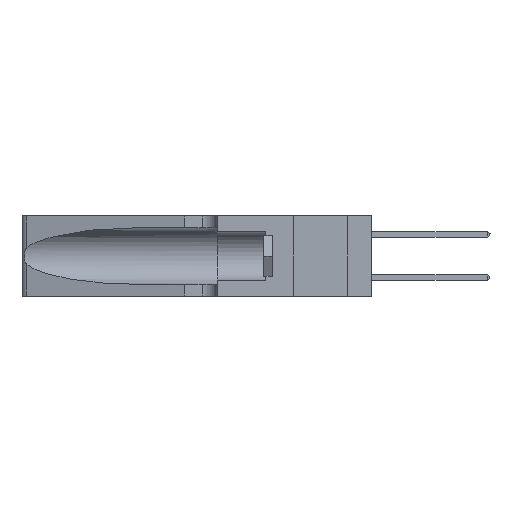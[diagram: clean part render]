
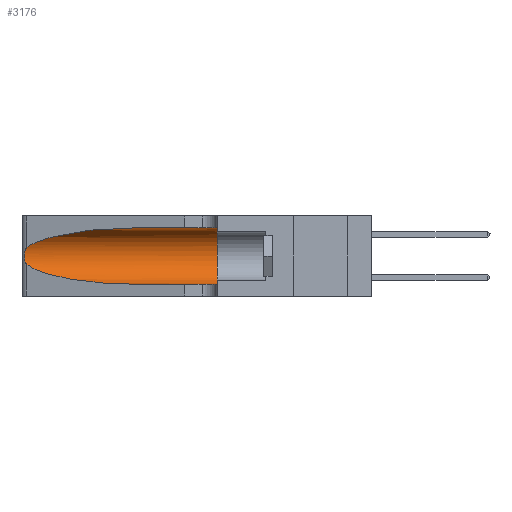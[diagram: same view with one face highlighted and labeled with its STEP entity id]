
A CAD part, left-side view. The second image highlights one B-rep face of the part: STEP entity #3176.
In plain terms, the highlighted cylindrical face has radius 3.308 mm (diameter 6.617 mm), a partial arc.
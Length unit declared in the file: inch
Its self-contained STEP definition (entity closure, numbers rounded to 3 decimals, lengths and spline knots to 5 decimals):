
#1540 = CARTESIAN_POINT ( 'NONE',  ( 0.25789, 1.23486, 0.15765 ) ) ;
#2517 = CARTESIAN_POINT ( 'NONE',  ( 0.1305, 1.61858, 0.185 ) ) ;
#3176 = ADVANCED_FACE ( 'NONE', ( #25702 ), #9307, .F. ) ;
#3346 =( BOUNDED_CURVE ( )  B_SPLINE_CURVE ( 3, ( #12811, #4509, #19047, #6638 ),
 .UNSPECIFIED., .F., .F. ) 
 B_SPLINE_CURVE_WITH_KNOTS ( ( 4, 4 ),
 ( 1.5708, 2.84003 ),
 .UNSPECIFIED. ) 
 CURVE ( )  GEOMETRIC_REPRESENTATION_ITEM ( )  RATIONAL_B_SPLINE_CURVE ( ( 1., 0.87, 0.87, 1. ) ) 
 REPRESENTATION_ITEM ( '' )  );
#3570 = CARTESIAN_POINT ( 'NONE',  ( 0.25487, 1.22718, 0.22369 ) ) ;
#3669 = CARTESIAN_POINT ( 'NONE',  ( 0.25555, 1.22993, 0.14849 ) ) ;
#4115 = VERTEX_POINT ( 'NONE', #24444 ) ;
#4509 = CARTESIAN_POINT ( 'NONE',  ( 0.18966, 0.96281, 0.31525 ) ) ;
#6603 = ORIENTED_EDGE ( 'NONE', *, *, #26753, .T. ) ;
#6638 = CARTESIAN_POINT ( 'NONE',  ( 0.25487, 1.22718, 0.22369 ) ) ;
#7506 = CARTESIAN_POINT ( 'NONE',  ( 0.25487, 1.22718, 0.14631 ) ) ;
#7804 = CARTESIAN_POINT ( 'NONE',  ( 0.25787, 1.23484, 0.2124 ) ) ;
#8794 = VERTEX_POINT ( 'NONE', #16846 ) ;
#9251 = EDGE_CURVE ( 'NONE', #15619, #22062, #12121, .T. ) ;
#9307 = CYLINDRICAL_SURFACE ( 'NONE', #14077, 0.13025 ) ;
#9560 = EDGE_CURVE ( 'NONE', #22062, #8794, #20831, .T. ) ;
#9878 = CARTESIAN_POINT ( 'NONE',  ( 0.26018, 1.23835, 0.19895 ) ) ;
#10433 = CARTESIAN_POINT ( 'NONE',  ( 0.18966, 0.96281, 0.05475 ) ) ;
#10836 = DIRECTION ( 'NONE',  ( 0., -1., 0. ) ) ;
#10981 = CARTESIAN_POINT ( 'NONE',  ( 0.1305, 1.61858, 0.05475 ) ) ;
#11306 = DIRECTION ( 'NONE',  ( 0., 1., 0. ) ) ;
#11959 = CARTESIAN_POINT ( 'NONE',  ( 0.26075, 1.23896, 0.178 ) ) ;
#12121 = LINE ( 'NONE', #22226, #17020 ) ;
#12380 = EDGE_LOOP ( 'NONE', ( #19701, #25297, #13927, #6603, #21835, #18582 ) ) ;
#12811 = CARTESIAN_POINT ( 'NONE',  ( 0.1305, 0.72297, 0.31525 ) ) ;
#13100 = DIRECTION ( 'NONE',  ( 0., -1., 0. ) ) ;
#13758 = VECTOR ( 'NONE', #13100, 39.37008 ) ;
#13927 = ORIENTED_EDGE ( 'NONE', *, *, #17995, .T. ) ;
#14077 = AXIS2_PLACEMENT_3D ( 'NONE', #2517, #10836, #25201 ) ;
#14095 = CARTESIAN_POINT ( 'NONE',  ( 0.25856, 1.23593, 0.16098 ) ) ;
#15213 = VERTEX_POINT ( 'NONE', #7506 ) ;
#15302 = VERTEX_POINT ( 'NONE', #26370 ) ;
#15619 = VERTEX_POINT ( 'NONE', #17568 ) ;
#15721 = CARTESIAN_POINT ( 'NONE',  ( 0.25555, 1.22994, 0.2215 ) ) ;
#16190 = CARTESIAN_POINT ( 'NONE',  ( 0.25639, 1.23186, 0.15144 ) ) ;
#16338 = CARTESIAN_POINT ( 'NONE',  ( 0.1305, 0.35, 0.31525 ) ) ;
#16846 = CARTESIAN_POINT ( 'NONE',  ( 0.1305, 0.35, 0.05475 ) ) ;
#17020 = VECTOR ( 'NONE', #24334, 39.37008 ) ;
#17568 = CARTESIAN_POINT ( 'NONE',  ( 0.1305, 0.72297, 0.31525 ) ) ;
#17995 = EDGE_CURVE ( 'NONE', #15213, #4115, #22595, .T. ) ;
#18224 = CARTESIAN_POINT ( 'NONE',  ( 0.25487, 1.22718, 0.14631 ) ) ;
#18582 = ORIENTED_EDGE ( 'NONE', *, *, #9251, .F. ) ;
#18606 = LINE ( 'NONE', #10981, #13758 ) ;
#18703 = CARTESIAN_POINT ( 'NONE',  ( 0.25487, 1.22718, 0.14631 ) ) ;
#19047 = CARTESIAN_POINT ( 'NONE',  ( 0.2373, 1.15595, 0.28018 ) ) ;
#19701 = ORIENTED_EDGE ( 'NONE', *, *, #21164, .T. ) ;
#20202 = CARTESIAN_POINT ( 'NONE',  ( 0.25639, 1.23184, 0.21858 ) ) ;
#20747 = CARTESIAN_POINT ( 'NONE',  ( 0.2373, 1.15595, 0.08982 ) ) ;
#20831 = CIRCLE ( 'NONE', #22224, 0.13025 ) ;
#21164 = EDGE_CURVE ( 'NONE', #15619, #15302, #3346, .T. ) ;
#21371 = EDGE_CURVE ( 'NONE', #15302, #15213, #25371, .T. ) ;
#21835 = ORIENTED_EDGE ( 'NONE', *, *, #9560, .F. ) ;
#22062 = VERTEX_POINT ( 'NONE', #16338 ) ;
#22224 = AXIS2_PLACEMENT_3D ( 'NONE', #23618, #11306, #25672 ) ;
#22226 = CARTESIAN_POINT ( 'NONE',  ( 0.1305, 1.61858, 0.31525 ) ) ;
#22233 = CARTESIAN_POINT ( 'NONE',  ( 0.25854, 1.2359, 0.20912 ) ) ;
#22595 =( BOUNDED_CURVE ( )  B_SPLINE_CURVE ( 3, ( #18703, #20747, #10433, #24823 ),
 .UNSPECIFIED., .F., .F. ) 
 B_SPLINE_CURVE_WITH_KNOTS ( ( 4, 4 ),
 ( 3.44316, 4.71239 ),
 .UNSPECIFIED. ) 
 CURVE ( )  GEOMETRIC_REPRESENTATION_ITEM ( )  RATIONAL_B_SPLINE_CURVE ( ( 1., 0.87, 0.87, 1. ) ) 
 REPRESENTATION_ITEM ( '' )  );
#23618 = CARTESIAN_POINT ( 'NONE',  ( 0.1305, 0.35, 0.185 ) ) ;
#24258 = CARTESIAN_POINT ( 'NONE',  ( 0.26075, 1.23896, 0.19203 ) ) ;
#24334 = DIRECTION ( 'NONE',  ( 0., -1., 0. ) ) ;
#24444 = CARTESIAN_POINT ( 'NONE',  ( 0.1305, 0.72297, 0.05475 ) ) ;
#24823 = CARTESIAN_POINT ( 'NONE',  ( 0.1305, 0.72297, 0.05475 ) ) ;
#25201 = DIRECTION ( 'NONE',  ( 0., 0., -1. ) ) ;
#25297 = ORIENTED_EDGE ( 'NONE', *, *, #21371, .T. ) ;
#25371 = B_SPLINE_CURVE_WITH_KNOTS ( 'NONE', 3,
 ( #3570, #15721, #20202, #7804, #22233, #9878, #24258, #11959, #26313, #14095, #1540, #16190, #3669, #18224 ),
 .UNSPECIFIED., .F., .F.,
 ( 4, 2, 2, 2, 2, 2, 4 ),
 ( 0., 0.00027, 0.00053, 0.00107, 0.0016, 0.00187, 0.00214 ),
 .UNSPECIFIED. ) ;
#25672 = DIRECTION ( 'NONE',  ( 0., 0., 1. ) ) ;
#25702 = FACE_OUTER_BOUND ( 'NONE', #12380, .T. ) ;
#26313 = CARTESIAN_POINT ( 'NONE',  ( 0.26017, 1.23833, 0.17102 ) ) ;
#26370 = CARTESIAN_POINT ( 'NONE',  ( 0.25487, 1.22718, 0.22369 ) ) ;
#26753 = EDGE_CURVE ( 'NONE', #4115, #8794, #18606, .T. ) ;
